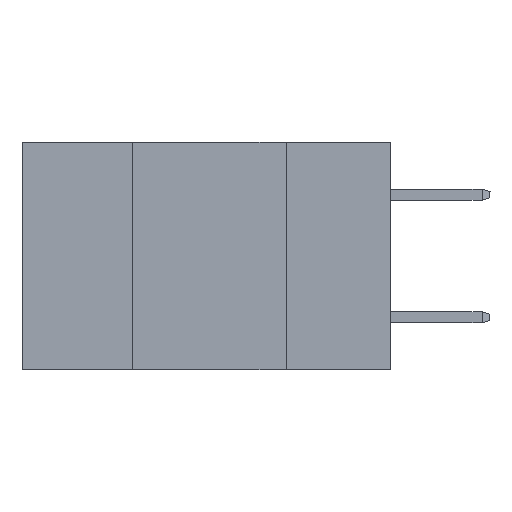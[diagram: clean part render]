
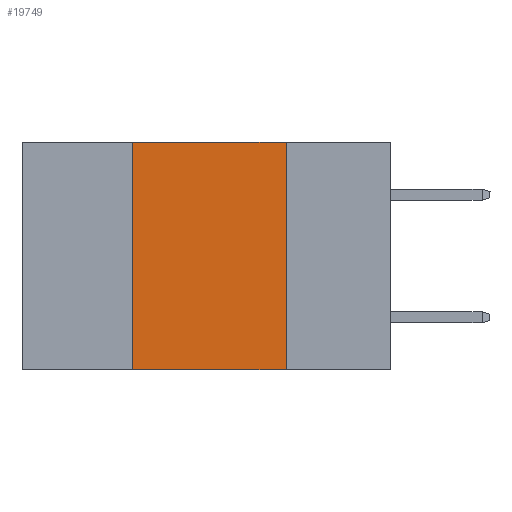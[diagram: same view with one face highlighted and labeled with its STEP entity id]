
A CAD part, left-side view. The second image highlights one B-rep face of the part: STEP entity #19749.
In plain terms, the highlighted planar face has unit normal (-1, 0, 0).
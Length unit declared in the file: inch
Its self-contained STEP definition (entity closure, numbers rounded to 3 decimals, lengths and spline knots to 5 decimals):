
#133 = DIRECTION ( 'NONE',  ( 1., 0., 0. ) ) ;
#274 = DIRECTION ( 'NONE',  ( 0., 0., -1. ) ) ;
#553 = LINE ( 'NONE', #9159, #26997 ) ;
#1272 = DIRECTION ( 'NONE',  ( 0., 0., -1. ) ) ;
#1472 = VECTOR ( 'NONE', #1272, 39.37008 ) ;
#1849 = ORIENTED_EDGE ( 'NONE', *, *, #8020, .F. ) ;
#3129 = LINE ( 'NONE', #9325, #1472 ) ;
#3502 = AXIS2_PLACEMENT_3D ( 'NONE', #25570, #133, #274 ) ;
#5195 = VERTEX_POINT ( 'NONE', #8673 ) ;
#6752 = VECTOR ( 'NONE', #19279, 39.37008 ) ;
#8020 = EDGE_CURVE ( 'NONE', #16870, #5195, #15227, .T. ) ;
#8180 = CARTESIAN_POINT ( 'NONE',  ( 0., 0.6, -0.37 ) ) ;
#8673 = CARTESIAN_POINT ( 'NONE',  ( 0., 0.42, 0. ) ) ;
#9088 = EDGE_CURVE ( 'NONE', #16610, #10265, #3129, .T. ) ;
#9159 = CARTESIAN_POINT ( 'NONE',  ( 0., 0.6, 0. ) ) ;
#9325 = CARTESIAN_POINT ( 'NONE',  ( 0., 0.17, 0. ) ) ;
#9896 = LINE ( 'NONE', #8180, #15786 ) ;
#10225 = EDGE_LOOP ( 'NONE', ( #23385, #14841, #1849, #14339 ) ) ;
#10265 = VERTEX_POINT ( 'NONE', #13160 ) ;
#13160 = CARTESIAN_POINT ( 'NONE',  ( 0., 0.17, -0.37 ) ) ;
#14244 = DIRECTION ( 'NONE',  ( 0., -1., 0. ) ) ;
#14339 = ORIENTED_EDGE ( 'NONE', *, *, #16154, .T. ) ;
#14841 = ORIENTED_EDGE ( 'NONE', *, *, #17300, .F. ) ;
#14926 = PLANE ( 'NONE',  #3502 ) ;
#15227 = LINE ( 'NONE', #15373, #6752 ) ;
#15373 = CARTESIAN_POINT ( 'NONE',  ( 0., 0.42, 0. ) ) ;
#15786 = VECTOR ( 'NONE', #14244, 39.37008 ) ;
#16106 = CARTESIAN_POINT ( 'NONE',  ( 0., 0.42, -0.37 ) ) ;
#16154 = EDGE_CURVE ( 'NONE', #16870, #10265, #9896, .T. ) ;
#16610 = VERTEX_POINT ( 'NONE', #25290 ) ;
#16870 = VERTEX_POINT ( 'NONE', #16106 ) ;
#17002 = FACE_OUTER_BOUND ( 'NONE', #10225, .T. ) ;
#17300 = EDGE_CURVE ( 'NONE', #5195, #16610, #553, .T. ) ;
#19279 = DIRECTION ( 'NONE',  ( 0., 0., 1. ) ) ;
#19749 = ADVANCED_FACE ( 'NONE', ( #17002 ), #14926, .F. ) ;
#23385 = ORIENTED_EDGE ( 'NONE', *, *, #9088, .F. ) ;
#25290 = CARTESIAN_POINT ( 'NONE',  ( 0., 0.17, 0. ) ) ;
#25570 = CARTESIAN_POINT ( 'NONE',  ( 0., 0.6, 0. ) ) ;
#26280 = DIRECTION ( 'NONE',  ( 0., -1., 0. ) ) ;
#26997 = VECTOR ( 'NONE', #26280, 39.37008 ) ;
